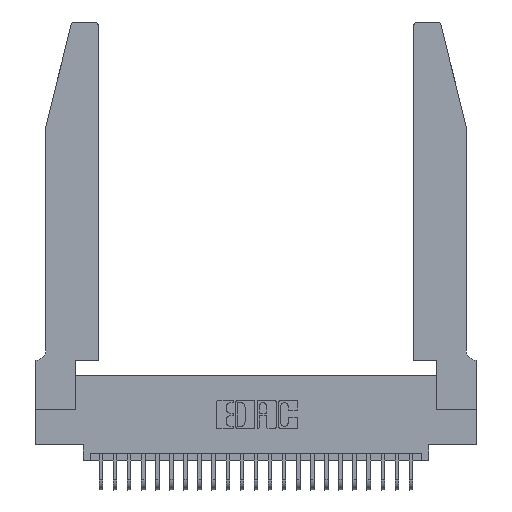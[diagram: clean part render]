
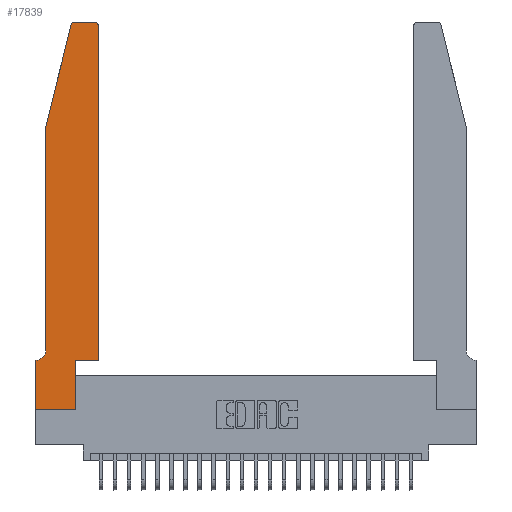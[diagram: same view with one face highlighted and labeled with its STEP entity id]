
A CAD part, top view. The second image highlights one B-rep face of the part: STEP entity #17839.
In plain terms, the highlighted planar face has unit normal (0, 0, 1).
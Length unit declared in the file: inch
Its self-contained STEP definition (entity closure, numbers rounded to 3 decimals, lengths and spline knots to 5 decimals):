
#91 = ORIENTED_EDGE ( 'NONE', *, *, #8951, .T. ) ;
#241 = VERTEX_POINT ( 'NONE', #5117 ) ;
#538 = VERTEX_POINT ( 'NONE', #9463 ) ;
#675 = CARTESIAN_POINT ( 'NONE',  ( 0., 0., 0.37 ) ) ;
#758 = CARTESIAN_POINT ( 'NONE',  ( 0.4505, 2.72, 0.37 ) ) ;
#810 = EDGE_CURVE ( 'NONE', #20482, #6466, #12622, .T. ) ;
#978 = AXIS2_PLACEMENT_3D ( 'NONE', #22237, #9843, #24281 ) ;
#1024 = CIRCLE ( 'NONE', #8176, 0.07 ) ;
#1783 = AXIS2_PLACEMENT_3D ( 'NONE', #4521, #19190, #6662 ) ;
#2106 = CARTESIAN_POINT ( 'NONE',  ( 0.2865, 0.35, 0.37 ) ) ;
#2206 = CARTESIAN_POINT ( 'NONE',  ( 0.2865, 0.35, 0.37 ) ) ;
#2213 = VECTOR ( 'NONE', #8073, 39.37008 ) ;
#2874 = DIRECTION ( 'NONE',  ( -1., 0., 0. ) ) ;
#3871 = VERTEX_POINT ( 'NONE', #758 ) ;
#3929 = ORIENTED_EDGE ( 'NONE', *, *, #27153, .T. ) ;
#4045 = CARTESIAN_POINT ( 'NONE',  ( 0., 0., 0.37 ) ) ;
#4396 = CARTESIAN_POINT ( 'NONE',  ( 0.284, 2.75, 0.37 ) ) ;
#4521 = CARTESIAN_POINT ( 'NONE',  ( 0.4205, 2.72, 0.37 ) ) ;
#4758 = ORIENTED_EDGE ( 'NONE', *, *, #13005, .T. ) ;
#5016 = VECTOR ( 'NONE', #12940, 39.37008 ) ;
#5117 = CARTESIAN_POINT ( 'NONE',  ( 0.0055, 0.35, 0.37 ) ) ;
#5624 = ORIENTED_EDGE ( 'NONE', *, *, #24084, .T. ) ;
#5666 = LINE ( 'NONE', #10792, #5016 ) ;
#5791 = CIRCLE ( 'NONE', #978, 0.03 ) ;
#6071 = VECTOR ( 'NONE', #9985, 39.37008 ) ;
#6128 = EDGE_LOOP ( 'NONE', ( #4758, #17677, #18698, #22600, #21871, #5624, #23067, #21463, #13145, #91, #16194, #3929 ) ) ;
#6466 = VERTEX_POINT ( 'NONE', #18389 ) ;
#6662 = DIRECTION ( 'NONE',  ( 1., 0., 0. ) ) ;
#6896 = CARTESIAN_POINT ( 'NONE',  ( 0., 0.35, 0.37 ) ) ;
#7005 = EDGE_CURVE ( 'NONE', #17595, #20703, #17310, .T. ) ;
#7765 = VERTEX_POINT ( 'NONE', #2206 ) ;
#8073 = DIRECTION ( 'NONE',  ( 0., 1., 0. ) ) ;
#8122 = PLANE ( 'NONE',  #11136 ) ;
#8176 = AXIS2_PLACEMENT_3D ( 'NONE', #22314, #9927, #24372 ) ;
#8676 = LINE ( 'NONE', #2106, #24561 ) ;
#8951 = EDGE_CURVE ( 'NONE', #7765, #20713, #12728, .T. ) ;
#9051 = VECTOR ( 'NONE', #22860, 39.37008 ) ;
#9421 = EDGE_CURVE ( 'NONE', #6466, #22364, #22944, .T. ) ;
#9463 = CARTESIAN_POINT ( 'NONE',  ( 0.4205, 2.75, 0.37 ) ) ;
#9534 = CIRCLE ( 'NONE', #1783, 0.03 ) ;
#9843 = DIRECTION ( 'NONE',  ( 0., 0., 1. ) ) ;
#9927 = DIRECTION ( 'NONE',  ( 0., 0., -1. ) ) ;
#9985 = DIRECTION ( 'NONE',  ( 1., 0., 0. ) ) ;
#10595 = DIRECTION ( 'NONE',  ( 0., 0., 1. ) ) ;
#10792 = CARTESIAN_POINT ( 'NONE',  ( 0.0755, 0.35, 0.37 ) ) ;
#10883 = EDGE_CURVE ( 'NONE', #18622, #17595, #14722, .T. ) ;
#11136 = AXIS2_PLACEMENT_3D ( 'NONE', #14760, #10595, #25021 ) ;
#11649 = VERTEX_POINT ( 'NONE', #4396 ) ;
#11817 = CARTESIAN_POINT ( 'NONE',  ( 0.25487, 2.72718, 0.37 ) ) ;
#11949 = LINE ( 'NONE', #17713, #12636 ) ;
#12102 = DIRECTION ( 'NONE',  ( 0., -1., 0. ) ) ;
#12503 = DIRECTION ( 'NONE',  ( 1., 0., 0. ) ) ;
#12622 = LINE ( 'NONE', #22928, #22872 ) ;
#12636 = VECTOR ( 'NONE', #2874, 39.37008 ) ;
#12728 = LINE ( 'NONE', #22708, #27108 ) ;
#12940 = DIRECTION ( 'NONE',  ( -1., 0., 0. ) ) ;
#13005 = EDGE_CURVE ( 'NONE', #538, #11649, #11949, .T. ) ;
#13145 = ORIENTED_EDGE ( 'NONE', *, *, #20790, .T. ) ;
#13290 = CARTESIAN_POINT ( 'NONE',  ( 0.0755, 0.42, 0.37 ) ) ;
#13641 = LINE ( 'NONE', #14544, #2213 ) ;
#14492 = FACE_OUTER_BOUND ( 'NONE', #6128, .T. ) ;
#14544 = CARTESIAN_POINT ( 'NONE',  ( 0.4505, 0.35, 0.37 ) ) ;
#14722 = LINE ( 'NONE', #4045, #9051 ) ;
#14760 = CARTESIAN_POINT ( 'NONE',  ( 0., 0.35, 0.37 ) ) ;
#16055 = EDGE_CURVE ( 'NONE', #22364, #241, #1024, .T. ) ;
#16194 = ORIENTED_EDGE ( 'NONE', *, *, #21785, .T. ) ;
#16723 = CARTESIAN_POINT ( 'NONE',  ( 0.2865, 0., 0.37 ) ) ;
#17310 = LINE ( 'NONE', #24434, #6071 ) ;
#17595 = VERTEX_POINT ( 'NONE', #675 ) ;
#17677 = ORIENTED_EDGE ( 'NONE', *, *, #17742, .T. ) ;
#17713 = CARTESIAN_POINT ( 'NONE',  ( 0.2605, 2.75, 0.37 ) ) ;
#17742 = EDGE_CURVE ( 'NONE', #11649, #20482, #5791, .T. ) ;
#17839 = ADVANCED_FACE ( 'NONE', ( #14492 ), #8122, .T. ) ;
#18389 = CARTESIAN_POINT ( 'NONE',  ( 0.0755, 2., 0.37 ) ) ;
#18622 = VERTEX_POINT ( 'NONE', #6896 ) ;
#18698 = ORIENTED_EDGE ( 'NONE', *, *, #810, .T. ) ;
#19019 = DIRECTION ( 'NONE',  ( 0., 1., 0. ) ) ;
#19190 = DIRECTION ( 'NONE',  ( 0., 0., 1. ) ) ;
#20482 = VERTEX_POINT ( 'NONE', #11817 ) ;
#20703 = VERTEX_POINT ( 'NONE', #16723 ) ;
#20713 = VERTEX_POINT ( 'NONE', #22853 ) ;
#20790 = EDGE_CURVE ( 'NONE', #20703, #7765, #8676, .T. ) ;
#21463 = ORIENTED_EDGE ( 'NONE', *, *, #7005, .T. ) ;
#21785 = EDGE_CURVE ( 'NONE', #20713, #3871, #13641, .T. ) ;
#21871 = ORIENTED_EDGE ( 'NONE', *, *, #16055, .T. ) ;
#22237 = CARTESIAN_POINT ( 'NONE',  ( 0.284, 2.72, 0.37 ) ) ;
#22305 = VECTOR ( 'NONE', #12102, 39.37008 ) ;
#22314 = CARTESIAN_POINT ( 'NONE',  ( 0.0055, 0.42, 0.37 ) ) ;
#22364 = VERTEX_POINT ( 'NONE', #13290 ) ;
#22600 = ORIENTED_EDGE ( 'NONE', *, *, #9421, .T. ) ;
#22708 = CARTESIAN_POINT ( 'NONE',  ( 0.4505, 0.35, 0.37 ) ) ;
#22853 = CARTESIAN_POINT ( 'NONE',  ( 0.4505, 0.35, 0.37 ) ) ;
#22860 = DIRECTION ( 'NONE',  ( 0., -1., 0. ) ) ;
#22872 = VECTOR ( 'NONE', #23077, 39.37008 ) ;
#22928 = CARTESIAN_POINT ( 'NONE',  ( 0.0755, 2., 0.37 ) ) ;
#22944 = LINE ( 'NONE', #24398, #22305 ) ;
#23067 = ORIENTED_EDGE ( 'NONE', *, *, #10883, .T. ) ;
#23077 = DIRECTION ( 'NONE',  ( -0.239, -0.971, 0. ) ) ;
#24084 = EDGE_CURVE ( 'NONE', #241, #18622, #5666, .T. ) ;
#24281 = DIRECTION ( 'NONE',  ( 1., 0., 0. ) ) ;
#24372 = DIRECTION ( 'NONE',  ( -1., 0., 0. ) ) ;
#24398 = CARTESIAN_POINT ( 'NONE',  ( 0.0755, 2., 0.37 ) ) ;
#24434 = CARTESIAN_POINT ( 'NONE',  ( 0., 0., 0.37 ) ) ;
#24561 = VECTOR ( 'NONE', #19019, 39.37008 ) ;
#25021 = DIRECTION ( 'NONE',  ( 1., 0., 0. ) ) ;
#27108 = VECTOR ( 'NONE', #12503, 39.37008 ) ;
#27153 = EDGE_CURVE ( 'NONE', #3871, #538, #9534, .T. ) ;
